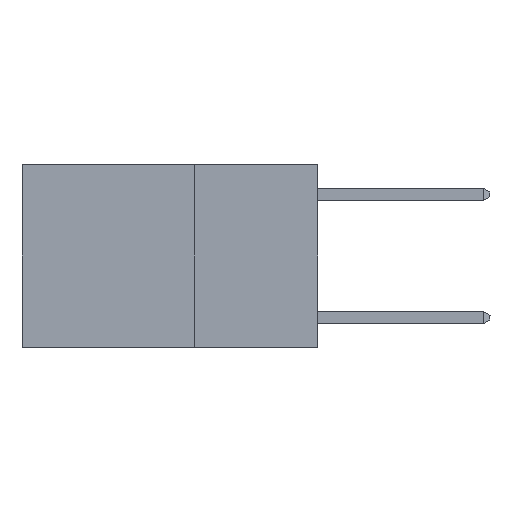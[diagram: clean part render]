
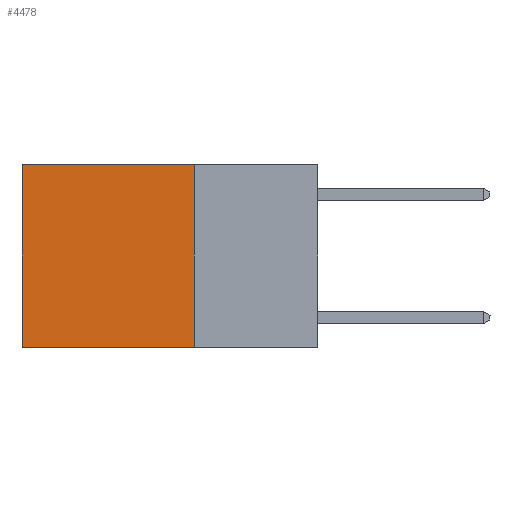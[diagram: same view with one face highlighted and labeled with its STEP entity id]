
A CAD part, left-side view. The second image highlights one B-rep face of the part: STEP entity #4478.
In plain terms, the highlighted planar face has unit normal (-1, 0, 0).
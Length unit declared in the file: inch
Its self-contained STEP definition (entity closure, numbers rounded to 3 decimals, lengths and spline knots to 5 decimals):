
#135 = LINE ( 'NONE', #9466, #7112 ) ;
#279 = FACE_OUTER_BOUND ( 'NONE', #9818, .T. ) ;
#983 = EDGE_CURVE ( 'NONE', #5682, #9451, #10472, .T. ) ;
#1216 = VECTOR ( 'NONE', #6796, 39.37008 ) ;
#1700 = DIRECTION ( 'NONE',  ( 0., 0., -1. ) ) ;
#2017 = ORIENTED_EDGE ( 'NONE', *, *, #3926, .F. ) ;
#2081 = PLANE ( 'NONE',  #10907 ) ;
#2213 = VERTEX_POINT ( 'NONE', #9389 ) ;
#2882 = LINE ( 'NONE', #6957, #7483 ) ;
#3068 = CARTESIAN_POINT ( 'NONE',  ( 0.2625, 0.6, -0.37 ) ) ;
#3911 = CARTESIAN_POINT ( 'NONE',  ( 0.2625, 0.25, 0. ) ) ;
#3926 = EDGE_CURVE ( 'NONE', #2213, #5130, #135, .T. ) ;
#4440 = DIRECTION ( 'NONE',  ( 0., 1., 0. ) ) ;
#4478 = ADVANCED_FACE ( 'NONE', ( #279 ), #2081, .F. ) ;
#4674 = CARTESIAN_POINT ( 'NONE',  ( 0.2625, 0.6, 0. ) ) ;
#4812 = DIRECTION ( 'NONE',  ( 0., 0., -1. ) ) ;
#4819 = EDGE_CURVE ( 'NONE', #5130, #9451, #2882, .T. ) ;
#5130 = VERTEX_POINT ( 'NONE', #9893 ) ;
#5424 = VECTOR ( 'NONE', #4440, 39.37008 ) ;
#5682 = VERTEX_POINT ( 'NONE', #4674 ) ;
#6439 = ORIENTED_EDGE ( 'NONE', *, *, #9038, .T. ) ;
#6770 = CARTESIAN_POINT ( 'NONE',  ( 0.2625, 0.6, 0. ) ) ;
#6796 = DIRECTION ( 'NONE',  ( 0., 0., -1. ) ) ;
#6957 = CARTESIAN_POINT ( 'NONE',  ( 0.2625, 0.25, -0.37 ) ) ;
#7112 = VECTOR ( 'NONE', #1700, 39.37008 ) ;
#7483 = VECTOR ( 'NONE', #7826, 39.37008 ) ;
#7826 = DIRECTION ( 'NONE',  ( 0., 1., 0. ) ) ;
#8896 = ORIENTED_EDGE ( 'NONE', *, *, #983, .T. ) ;
#9038 = EDGE_CURVE ( 'NONE', #2213, #5682, #9900, .T. ) ;
#9389 = CARTESIAN_POINT ( 'NONE',  ( 0.2625, 0.25, 0. ) ) ;
#9451 = VERTEX_POINT ( 'NONE', #3068 ) ;
#9466 = CARTESIAN_POINT ( 'NONE',  ( 0.2625, 0.25, 0. ) ) ;
#9818 = EDGE_LOOP ( 'NONE', ( #8896, #10623, #2017, #6439 ) ) ;
#9874 = DIRECTION ( 'NONE',  ( 1., 0., 0. ) ) ;
#9893 = CARTESIAN_POINT ( 'NONE',  ( 0.2625, 0.25, -0.37 ) ) ;
#9900 = LINE ( 'NONE', #11153, #5424 ) ;
#10472 = LINE ( 'NONE', #6770, #1216 ) ;
#10623 = ORIENTED_EDGE ( 'NONE', *, *, #4819, .F. ) ;
#10907 = AXIS2_PLACEMENT_3D ( 'NONE', #3911, #9874, #4812 ) ;
#11153 = CARTESIAN_POINT ( 'NONE',  ( 0.2625, 0.25, 0. ) ) ;
